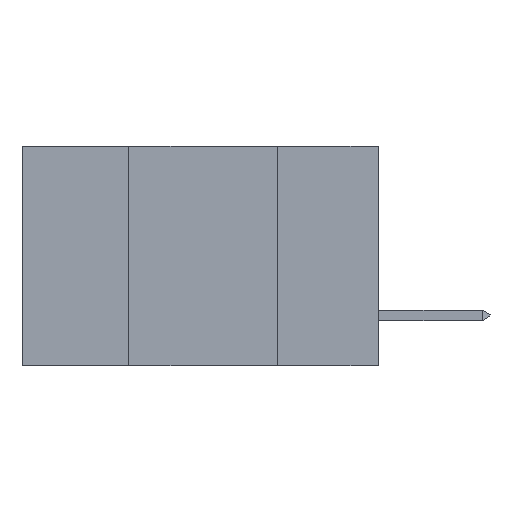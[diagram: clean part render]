
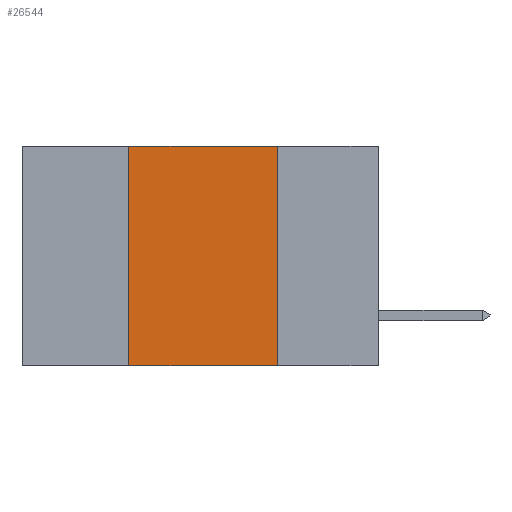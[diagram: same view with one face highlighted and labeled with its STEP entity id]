
A CAD part, left-side view. The second image highlights one B-rep face of the part: STEP entity #26544.
In plain terms, the highlighted planar face has unit normal (-1, 0, 0).
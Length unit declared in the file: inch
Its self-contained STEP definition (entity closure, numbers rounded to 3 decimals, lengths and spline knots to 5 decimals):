
#2181 = LINE ( 'NONE', #22228, #19747 ) ;
#2287 = VECTOR ( 'NONE', #22339, 39.37008 ) ;
#5028 = EDGE_LOOP ( 'NONE', ( #9442, #21389, #9407, #26639 ) ) ;
#7170 = DIRECTION ( 'NONE',  ( 0., -1., 0. ) ) ;
#8102 = DIRECTION ( 'NONE',  ( 0., 0., 1. ) ) ;
#8201 = CARTESIAN_POINT ( 'NONE',  ( 0., 0.42, 0. ) ) ;
#8339 = VERTEX_POINT ( 'NONE', #23485 ) ;
#8459 = LINE ( 'NONE', #26777, #2287 ) ;
#9407 = ORIENTED_EDGE ( 'NONE', *, *, #22826, .F. ) ;
#9442 = ORIENTED_EDGE ( 'NONE', *, *, #24346, .F. ) ;
#9984 = PLANE ( 'NONE',  #26224 ) ;
#11025 = FACE_OUTER_BOUND ( 'NONE', #5028, .T. ) ;
#12304 = DIRECTION ( 'NONE',  ( 1., 0., 0. ) ) ;
#12887 = VERTEX_POINT ( 'NONE', #28087 ) ;
#13855 = CARTESIAN_POINT ( 'NONE',  ( 0., 0.42, -0.37 ) ) ;
#15460 = DIRECTION ( 'NONE',  ( 0., -1., 0. ) ) ;
#16267 = LINE ( 'NONE', #20809, #27512 ) ;
#17157 = LINE ( 'NONE', #8201, #28418 ) ;
#19747 = VECTOR ( 'NONE', #15460, 39.37008 ) ;
#19778 = EDGE_CURVE ( 'NONE', #27697, #21269, #2181, .T. ) ;
#20561 = EDGE_CURVE ( 'NONE', #12887, #8339, #16267, .T. ) ;
#20809 = CARTESIAN_POINT ( 'NONE',  ( 0., 0.6, 0. ) ) ;
#21269 = VERTEX_POINT ( 'NONE', #27792 ) ;
#21389 = ORIENTED_EDGE ( 'NONE', *, *, #20561, .F. ) ;
#22228 = CARTESIAN_POINT ( 'NONE',  ( 0., 0.6, -0.37 ) ) ;
#22339 = DIRECTION ( 'NONE',  ( 0., 0., -1. ) ) ;
#22826 = EDGE_CURVE ( 'NONE', #27697, #12887, #17157, .T. ) ;
#23485 = CARTESIAN_POINT ( 'NONE',  ( 0., 0.17, 0. ) ) ;
#24346 = EDGE_CURVE ( 'NONE', #8339, #21269, #8459, .T. ) ;
#25878 = CARTESIAN_POINT ( 'NONE',  ( 0., 0.6, 0. ) ) ;
#26224 = AXIS2_PLACEMENT_3D ( 'NONE', #25878, #12304, #28126 ) ;
#26544 = ADVANCED_FACE ( 'NONE', ( #11025 ), #9984, .F. ) ;
#26639 = ORIENTED_EDGE ( 'NONE', *, *, #19778, .T. ) ;
#26777 = CARTESIAN_POINT ( 'NONE',  ( 0., 0.17, 0. ) ) ;
#27512 = VECTOR ( 'NONE', #7170, 39.37008 ) ;
#27697 = VERTEX_POINT ( 'NONE', #13855 ) ;
#27792 = CARTESIAN_POINT ( 'NONE',  ( 0., 0.17, -0.37 ) ) ;
#28087 = CARTESIAN_POINT ( 'NONE',  ( 0., 0.42, 0. ) ) ;
#28126 = DIRECTION ( 'NONE',  ( 0., 0., -1. ) ) ;
#28418 = VECTOR ( 'NONE', #8102, 39.37008 ) ;
